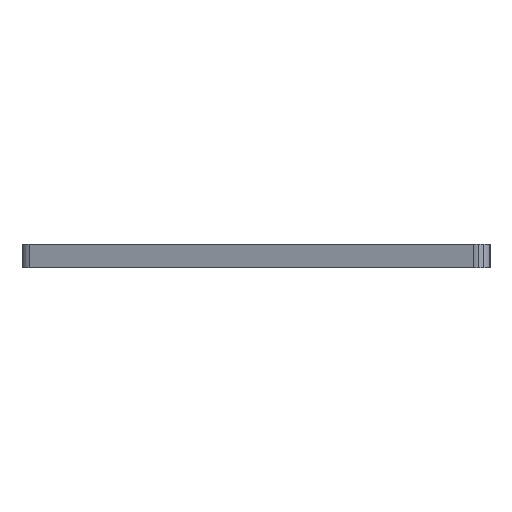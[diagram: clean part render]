
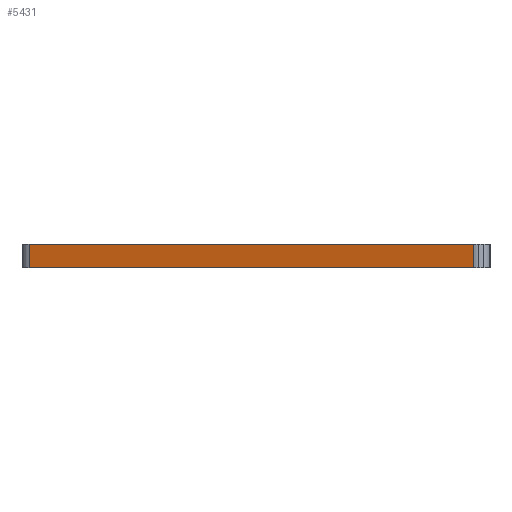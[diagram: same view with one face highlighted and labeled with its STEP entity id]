
A CAD part, left-side view. The second image highlights one B-rep face of the part: STEP entity #5431.
In plain terms, the highlighted planar face has unit normal (-0.957, 0.29, 0).
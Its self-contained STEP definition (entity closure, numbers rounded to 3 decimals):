
#473 = FACE_OUTER_BOUND ( 'NONE', #6066, .T. ) ;
#744 = VERTEX_POINT ( 'NONE', #4905 ) ;
#813 = CARTESIAN_POINT ( 'NONE',  ( -110.636, -18.441, 0.203 ) ) ;
#916 = DIRECTION ( 'NONE',  ( 0., 0., -1. ) ) ;
#1094 = CARTESIAN_POINT ( 'NONE',  ( -110.636, -18.441, 0.203 ) ) ;
#1341 = DIRECTION ( 'NONE',  ( 0.957, -0.29, 0. ) ) ;
#1651 = DIRECTION ( 'NONE',  ( -0.29, -0.957, 0. ) ) ;
#1655 = ORIENTED_EDGE ( 'NONE', *, *, #5173, .F. ) ;
#1770 = VECTOR ( 'NONE', #3363, 1000. ) ;
#1979 = CARTESIAN_POINT ( 'NONE',  ( -111.816, -22.34, 0. ) ) ;
#2067 = VERTEX_POINT ( 'NONE', #2886 ) ;
#2096 = ORIENTED_EDGE ( 'NONE', *, *, #3455, .T. ) ;
#2271 = VECTOR ( 'NONE', #4116, 1000. ) ;
#2324 = ORIENTED_EDGE ( 'NONE', *, *, #3530, .F. ) ;
#2423 = VECTOR ( 'NONE', #1651, 1000. ) ;
#2643 = ORIENTED_EDGE ( 'NONE', *, *, #5705, .T. ) ;
#2886 = CARTESIAN_POINT ( 'NONE',  ( -110.636, -18.441, 0.203 ) ) ;
#3196 = AXIS2_PLACEMENT_3D ( 'NONE', #813, #1341, #4856 ) ;
#3363 = DIRECTION ( 'NONE',  ( 0., 0., -1. ) ) ;
#3455 = EDGE_CURVE ( 'NONE', #2067, #4591, #5591, .T. ) ;
#3469 = CARTESIAN_POINT ( 'NONE',  ( -110.636, -18.441, 0. ) ) ;
#3530 = EDGE_CURVE ( 'NONE', #744, #3894, #5293, .T. ) ;
#3741 = LINE ( 'NONE', #5136, #2423 ) ;
#3894 = VERTEX_POINT ( 'NONE', #1979 ) ;
#4116 = DIRECTION ( 'NONE',  ( -0.29, -0.957, 0. ) ) ;
#4591 = VERTEX_POINT ( 'NONE', #3469 ) ;
#4856 = DIRECTION ( 'NONE',  ( 0.29, 0.957, 0. ) ) ;
#4905 = CARTESIAN_POINT ( 'NONE',  ( -111.816, -22.34, 0.203 ) ) ;
#4940 = CARTESIAN_POINT ( 'NONE',  ( -111.816, -22.34, 0.203 ) ) ;
#5089 = LINE ( 'NONE', #1094, #2271 ) ;
#5130 = VECTOR ( 'NONE', #916, 1000. ) ;
#5136 = CARTESIAN_POINT ( 'NONE',  ( -110.636, -18.441, 0. ) ) ;
#5173 = EDGE_CURVE ( 'NONE', #2067, #744, #5089, .T. ) ;
#5293 = LINE ( 'NONE', #4940, #5130 ) ;
#5431 = ADVANCED_FACE ( 'NONE', ( #473 ), #5831, .F. ) ;
#5591 = LINE ( 'NONE', #5873, #1770 ) ;
#5705 = EDGE_CURVE ( 'NONE', #4591, #3894, #3741, .T. ) ;
#5831 = PLANE ( 'NONE',  #3196 ) ;
#5873 = CARTESIAN_POINT ( 'NONE',  ( -110.636, -18.441, 0.203 ) ) ;
#6066 = EDGE_LOOP ( 'NONE', ( #2643, #2324, #1655, #2096 ) ) ;
